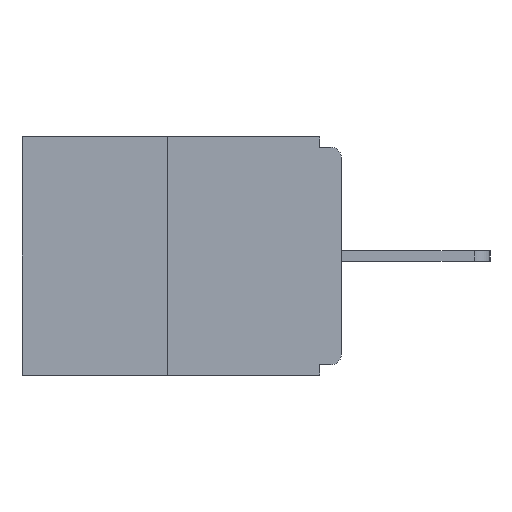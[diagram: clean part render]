
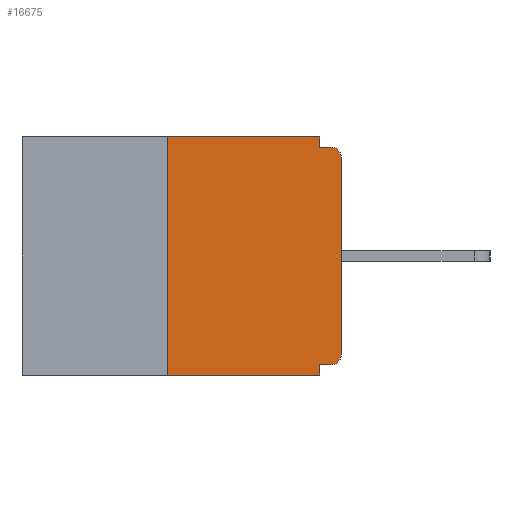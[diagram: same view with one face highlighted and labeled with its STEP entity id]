
A CAD part, left-side view. The second image highlights one B-rep face of the part: STEP entity #16675.
In plain terms, the highlighted planar face has unit normal (-1, 0, 0).
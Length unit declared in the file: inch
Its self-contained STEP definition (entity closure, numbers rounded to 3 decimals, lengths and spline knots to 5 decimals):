
#56 = CARTESIAN_POINT ( 'NONE',  ( 0., 0.015, -0.015 ) ) ;
#88 = DIRECTION ( 'NONE',  ( 0., 0., -1. ) ) ;
#817 = AXIS2_PLACEMENT_3D ( 'NONE', #12601, #18987, #24957 ) ;
#1263 = VERTEX_POINT ( 'NONE', #10821 ) ;
#1475 = AXIS2_PLACEMENT_3D ( 'NONE', #17043, #25645, #88 ) ;
#1674 = ORIENTED_EDGE ( 'NONE', *, *, #19798, .F. ) ;
#1694 = VERTEX_POINT ( 'NONE', #6858 ) ;
#2075 = CARTESIAN_POINT ( 'NONE',  ( 0., 0.031, -0.343 ) ) ;
#2640 = FACE_OUTER_BOUND ( 'NONE', #21806, .T. ) ;
#2770 = EDGE_CURVE ( 'NONE', #1263, #19018, #18597, .T. ) ;
#3093 = VERTEX_POINT ( 'NONE', #19813 ) ;
#3562 = VERTEX_POINT ( 'NONE', #22243 ) ;
#3753 = CARTESIAN_POINT ( 'NONE',  ( 0., 0., 0. ) ) ;
#3835 = CARTESIAN_POINT ( 'NONE',  ( 0., 0., -0.313 ) ) ;
#3984 = EDGE_CURVE ( 'NONE', #18679, #21951, #18448, .T. ) ;
#4284 = EDGE_CURVE ( 'NONE', #7685, #3093, #17595, .T. ) ;
#4828 = CARTESIAN_POINT ( 'NONE',  ( 0., 0.031, -0.328 ) ) ;
#5103 = CARTESIAN_POINT ( 'NONE',  ( 0., 0.25, 0. ) ) ;
#5606 = ORIENTED_EDGE ( 'NONE', *, *, #6074, .T. ) ;
#5699 = LINE ( 'NONE', #2075, #27381 ) ;
#6074 = EDGE_CURVE ( 'NONE', #3562, #17452, #9924, .T. ) ;
#6097 = ORIENTED_EDGE ( 'NONE', *, *, #11421, .T. ) ;
#6204 = EDGE_CURVE ( 'NONE', #21951, #7685, #15655, .T. ) ;
#6858 = CARTESIAN_POINT ( 'NONE',  ( 0., 0.031, -0.343 ) ) ;
#6899 = DIRECTION ( 'NONE',  ( 0., -1., 0. ) ) ;
#7520 = ORIENTED_EDGE ( 'NONE', *, *, #12031, .F. ) ;
#7685 = VERTEX_POINT ( 'NONE', #25382 ) ;
#7926 = ORIENTED_EDGE ( 'NONE', *, *, #25150, .F. ) ;
#8384 = DIRECTION ( 'NONE',  ( 0., -1., 0. ) ) ;
#9924 = CIRCLE ( 'NONE', #1475, 0.015 ) ;
#10157 = DIRECTION ( 'NONE',  ( 0., 0., 1. ) ) ;
#10515 = EDGE_CURVE ( 'NONE', #17452, #1263, #22513, .T. ) ;
#10821 = CARTESIAN_POINT ( 'NONE',  ( 0., 0., -0.03 ) ) ;
#11421 = EDGE_CURVE ( 'NONE', #18679, #1694, #23245, .T. ) ;
#11528 = DIRECTION ( 'NONE',  ( 0., 0., -1. ) ) ;
#12013 = DIRECTION ( 'NONE',  ( 0., -1., 0. ) ) ;
#12031 = EDGE_CURVE ( 'NONE', #3562, #21293, #18037, .T. ) ;
#12601 = CARTESIAN_POINT ( 'NONE',  ( 0., 0.015, -0.03 ) ) ;
#12645 = DIRECTION ( 'NONE',  ( 0., 0., -1. ) ) ;
#13427 = CARTESIAN_POINT ( 'NONE',  ( 0., 0.031, 0. ) ) ;
#13818 = LINE ( 'NONE', #26585, #22710 ) ;
#15635 = ORIENTED_EDGE ( 'NONE', *, *, #3984, .F. ) ;
#15655 = LINE ( 'NONE', #26196, #22330 ) ;
#15772 = ORIENTED_EDGE ( 'NONE', *, *, #4284, .F. ) ;
#15811 = ORIENTED_EDGE ( 'NONE', *, *, #10515, .T. ) ;
#15822 = CARTESIAN_POINT ( 'NONE',  ( 0., 0., -0.328 ) ) ;
#16675 = ADVANCED_FACE ( 'NONE', ( #2640 ), #21825, .F. ) ;
#17043 = CARTESIAN_POINT ( 'NONE',  ( 0., 0.015, -0.313 ) ) ;
#17113 = CARTESIAN_POINT ( 'NONE',  ( 0., 0.25, 0. ) ) ;
#17151 = VECTOR ( 'NONE', #8384, 39.37008 ) ;
#17452 = VERTEX_POINT ( 'NONE', #3835 ) ;
#17595 = LINE ( 'NONE', #13427, #19562 ) ;
#18037 = LINE ( 'NONE', #15822, #26071 ) ;
#18448 = LINE ( 'NONE', #5103, #26168 ) ;
#18597 = CIRCLE ( 'NONE', #817, 0.015 ) ;
#18679 = VERTEX_POINT ( 'NONE', #23017 ) ;
#18987 = DIRECTION ( 'NONE',  ( -1., 0., 0. ) ) ;
#19018 = VERTEX_POINT ( 'NONE', #56 ) ;
#19562 = VECTOR ( 'NONE', #21910, 39.37008 ) ;
#19798 = EDGE_CURVE ( 'NONE', #21293, #1694, #5699, .T. ) ;
#19813 = CARTESIAN_POINT ( 'NONE',  ( 0., 0.031, -0.015 ) ) ;
#19867 = DIRECTION ( 'NONE',  ( 1., 0., 0. ) ) ;
#21293 = VERTEX_POINT ( 'NONE', #4828 ) ;
#21410 = AXIS2_PLACEMENT_3D ( 'NONE', #25969, #19867, #11528 ) ;
#21806 = EDGE_LOOP ( 'NONE', ( #22799, #15635, #6097, #1674, #7520, #5606, #15811, #26613, #7926, #15772 ) ) ;
#21825 = PLANE ( 'NONE',  #21410 ) ;
#21910 = DIRECTION ( 'NONE',  ( 0., 0., -1. ) ) ;
#21951 = VERTEX_POINT ( 'NONE', #17113 ) ;
#22243 = CARTESIAN_POINT ( 'NONE',  ( 0., 0.015, -0.328 ) ) ;
#22330 = VECTOR ( 'NONE', #6899, 39.37008 ) ;
#22355 = DIRECTION ( 'NONE',  ( 0., 0., 1. ) ) ;
#22513 = LINE ( 'NONE', #3753, #22864 ) ;
#22710 = VECTOR ( 'NONE', #12013, 39.37008 ) ;
#22799 = ORIENTED_EDGE ( 'NONE', *, *, #6204, .F. ) ;
#22864 = VECTOR ( 'NONE', #10157, 39.37008 ) ;
#23017 = CARTESIAN_POINT ( 'NONE',  ( 0., 0.25, -0.343 ) ) ;
#23245 = LINE ( 'NONE', #25718, #17151 ) ;
#24957 = DIRECTION ( 'NONE',  ( 0., 0., -1. ) ) ;
#25150 = EDGE_CURVE ( 'NONE', #3093, #19018, #13818, .T. ) ;
#25382 = CARTESIAN_POINT ( 'NONE',  ( 0., 0.031, 0. ) ) ;
#25645 = DIRECTION ( 'NONE',  ( -1., 0., 0. ) ) ;
#25718 = CARTESIAN_POINT ( 'NONE',  ( 0., 0.46, -0.343 ) ) ;
#25969 = CARTESIAN_POINT ( 'NONE',  ( 0., 0.46, 0. ) ) ;
#26071 = VECTOR ( 'NONE', #26504, 39.37008 ) ;
#26168 = VECTOR ( 'NONE', #22355, 39.37008 ) ;
#26196 = CARTESIAN_POINT ( 'NONE',  ( 0., 0.46, 0. ) ) ;
#26504 = DIRECTION ( 'NONE',  ( 0., 1., 0. ) ) ;
#26585 = CARTESIAN_POINT ( 'NONE',  ( 0., 0., -0.015 ) ) ;
#26613 = ORIENTED_EDGE ( 'NONE', *, *, #2770, .T. ) ;
#27381 = VECTOR ( 'NONE', #12645, 39.37008 ) ;
